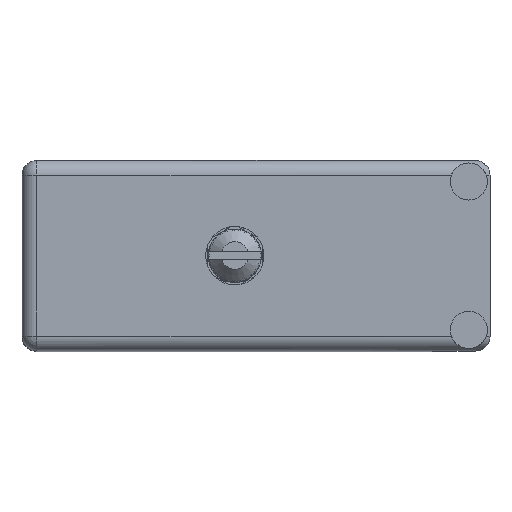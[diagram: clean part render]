
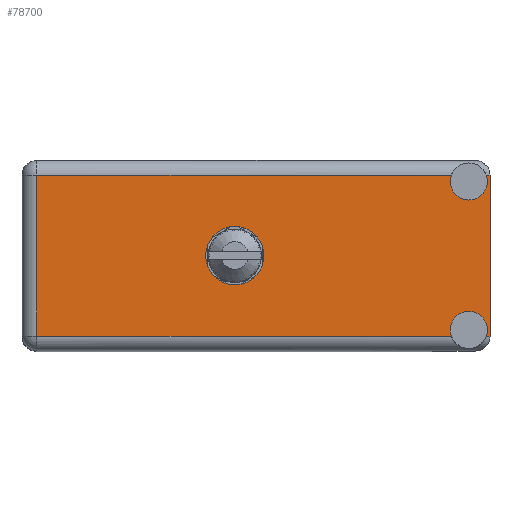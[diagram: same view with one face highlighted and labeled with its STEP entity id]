
A CAD part, top view. The second image highlights one B-rep face of the part: STEP entity #78700.
In plain terms, the highlighted face is planar.
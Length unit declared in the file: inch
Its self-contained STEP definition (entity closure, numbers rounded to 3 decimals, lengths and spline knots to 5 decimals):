
#2016 = EDGE_CURVE ( 'NONE', #110366, #90084, #36527, .T. ) ;
#2935 = CARTESIAN_POINT ( 'NONE',  ( 1.004, 1.566, -0.4495 ) ) ;
#3566 = CARTESIAN_POINT ( 'NONE',  ( 2.208, 1.566, -0.07 ) ) ;
#3950 = DIRECTION ( 'NONE',  ( 0., 1., 0. ) ) ;
#4356 = VERTEX_POINT ( 'NONE', #86213 ) ;
#5096 = ORIENTED_EDGE ( 'NONE', *, *, #92905, .T. ) ;
#5624 = EDGE_LOOP ( 'NONE', ( #109971, #22260, #44195, #107811, #81804, #33854, #102576, #89367, #27568, #5096 ) ) ;
#7193 = CARTESIAN_POINT ( 'NONE',  ( 2.19038, 1.566, -0.07 ) ) ;
#8008 = VERTEX_POINT ( 'NONE', #30675 ) ;
#9982 = CARTESIAN_POINT ( 'NONE',  ( 0., 1.566, -0.829 ) ) ;
#11879 = DIRECTION ( 'NONE',  ( 0., 0., 1. ) ) ;
#13929 = CARTESIAN_POINT ( 'NONE',  ( 0.07, 1.566, -0.07 ) ) ;
#14303 = VERTEX_POINT ( 'NONE', #78402 ) ;
#14353 = CARTESIAN_POINT ( 'NONE',  ( 2.208, 1.566, -0.07 ) ) ;
#14732 = VERTEX_POINT ( 'NONE', #71281 ) ;
#14805 = CARTESIAN_POINT ( 'NONE',  ( 0.07, 1.566, -0.829 ) ) ;
#18191 = CARTESIAN_POINT ( 'NONE',  ( 1.004, 1.566, -0.312 ) ) ;
#18658 = CIRCLE ( 'NONE', #94053, 0.0875 ) ;
#19000 = EDGE_CURVE ( 'NONE', #14303, #85294, #23795, .T. ) ;
#19820 = AXIS2_PLACEMENT_3D ( 'NONE', #71163, #61819, #53638 ) ;
#22245 = EDGE_CURVE ( 'NONE', #14732, #39829, #66998, .T. ) ;
#22260 = ORIENTED_EDGE ( 'NONE', *, *, #31615, .F. ) ;
#23795 = CIRCLE ( 'NONE', #19820, 0.1375 ) ;
#24312 = CIRCLE ( 'NONE', #114780, 0.0875 ) ;
#26989 = CARTESIAN_POINT ( 'NONE',  ( 2.108, 1.566, -0.0995 ) ) ;
#27568 = ORIENTED_EDGE ( 'NONE', *, *, #2016, .T. ) ;
#28002 = CARTESIAN_POINT ( 'NONE',  ( 2.108, 1.566, -0.0995 ) ) ;
#28774 = DIRECTION ( 'NONE',  ( 0., 0., 1. ) ) ;
#29146 = LINE ( 'NONE', #3566, #103081 ) ;
#29186 = EDGE_CURVE ( 'NONE', #110366, #4356, #18658, .T. ) ;
#30675 = CARTESIAN_POINT ( 'NONE',  ( 2.108, 1.566, -0.187 ) ) ;
#30737 = CARTESIAN_POINT ( 'NONE',  ( 2.02562, 1.566, -0.829 ) ) ;
#31615 = EDGE_CURVE ( 'NONE', #8008, #68920, #24312, .T. ) ;
#33402 = CARTESIAN_POINT ( 'NONE',  ( 2.02562, 1.566, -0.07 ) ) ;
#33520 = DIRECTION ( 'NONE',  ( 1., 0., 0. ) ) ;
#33854 = ORIENTED_EDGE ( 'NONE', *, *, #22245, .T. ) ;
#35209 = DIRECTION ( 'NONE',  ( 0., 0., 1. ) ) ;
#35634 = DIRECTION ( 'NONE',  ( -1., 0., 0. ) ) ;
#36142 = EDGE_LOOP ( 'NONE', ( #79937, #96858 ) ) ;
#36356 = CARTESIAN_POINT ( 'NONE',  ( 2.208, 1.566, 0. ) ) ;
#36527 = LINE ( 'NONE', #9982, #104851 ) ;
#38029 = LINE ( 'NONE', #82446, #76975 ) ;
#39829 = VERTEX_POINT ( 'NONE', #103362 ) ;
#44177 = CARTESIAN_POINT ( 'NONE',  ( 2.108, 1.566, -0.7995 ) ) ;
#44195 = ORIENTED_EDGE ( 'NONE', *, *, #73581, .F. ) ;
#48921 = LINE ( 'NONE', #61186, #107485 ) ;
#50059 = DIRECTION ( 'NONE',  ( 0., 0., 1. ) ) ;
#51718 = VECTOR ( 'NONE', #58402, 39.37008 ) ;
#53400 = CIRCLE ( 'NONE', #66712, 0.0875 ) ;
#53638 = DIRECTION ( 'NONE',  ( 0., 0., 1. ) ) ;
#53927 = DIRECTION ( 'NONE',  ( 0., 0., 1. ) ) ;
#58402 = DIRECTION ( 'NONE',  ( -1., 0., 0. ) ) ;
#58977 = CIRCLE ( 'NONE', #114504, 0.1375 ) ;
#59398 = DIRECTION ( 'NONE',  ( 0., 1., 0. ) ) ;
#61186 = CARTESIAN_POINT ( 'NONE',  ( 2.208, 1.566, -0.07 ) ) ;
#61330 = DIRECTION ( 'NONE',  ( 0., 0., 1. ) ) ;
#61819 = DIRECTION ( 'NONE',  ( 0., 1., 0. ) ) ;
#63246 = DIRECTION ( 'NONE',  ( 0., 1., 0. ) ) ;
#64933 = FACE_BOUND ( 'NONE', #36142, .T. ) ;
#66712 = AXIS2_PLACEMENT_3D ( 'NONE', #44177, #107260, #61330 ) ;
#66998 = LINE ( 'NONE', #109500, #51718 ) ;
#68920 = VERTEX_POINT ( 'NONE', #33402 ) ;
#70674 = DIRECTION ( 'NONE',  ( 0., 0., 1. ) ) ;
#71163 = CARTESIAN_POINT ( 'NONE',  ( 1.004, 1.566, -0.4495 ) ) ;
#71281 = CARTESIAN_POINT ( 'NONE',  ( 2.208, 1.566, -0.829 ) ) ;
#73581 = EDGE_CURVE ( 'NONE', #88315, #8008, #78982, .T. ) ;
#74115 = VERTEX_POINT ( 'NONE', #14353 ) ;
#76975 = VECTOR ( 'NONE', #81665, 39.37008 ) ;
#77280 = CARTESIAN_POINT ( 'NONE',  ( 0., 1.566, -0.899 ) ) ;
#78402 = CARTESIAN_POINT ( 'NONE',  ( 1.004, 1.566, -0.587 ) ) ;
#78700 = ADVANCED_FACE ( 'NONE', ( #64933, #99868 ), #111615, .T. ) ;
#78982 = CIRCLE ( 'NONE', #91266, 0.0875 ) ;
#79937 = ORIENTED_EDGE ( 'NONE', *, *, #109669, .F. ) ;
#80832 = AXIS2_PLACEMENT_3D ( 'NONE', #77280, #59398, #50059 ) ;
#81665 = DIRECTION ( 'NONE',  ( 0., 0., 1. ) ) ;
#81804 = ORIENTED_EDGE ( 'NONE', *, *, #109503, .F. ) ;
#82446 = CARTESIAN_POINT ( 'NONE',  ( 0.07, 1.566, -0.899 ) ) ;
#82676 = LINE ( 'NONE', #36356, #109188 ) ;
#85294 = VERTEX_POINT ( 'NONE', #18191 ) ;
#86073 = EDGE_CURVE ( 'NONE', #88315, #74115, #29146, .T. ) ;
#86213 = CARTESIAN_POINT ( 'NONE',  ( 2.108, 1.566, -0.712 ) ) ;
#88315 = VERTEX_POINT ( 'NONE', #7193 ) ;
#89157 = VERTEX_POINT ( 'NONE', #13929 ) ;
#89367 = ORIENTED_EDGE ( 'NONE', *, *, #29186, .F. ) ;
#90084 = VERTEX_POINT ( 'NONE', #14805 ) ;
#91266 = AXIS2_PLACEMENT_3D ( 'NONE', #28002, #3950, #28774 ) ;
#92905 = EDGE_CURVE ( 'NONE', #90084, #89157, #38029, .T. ) ;
#94053 = AXIS2_PLACEMENT_3D ( 'NONE', #106139, #106525, #35209 ) ;
#96858 = ORIENTED_EDGE ( 'NONE', *, *, #19000, .F. ) ;
#99868 = FACE_OUTER_BOUND ( 'NONE', #5624, .T. ) ;
#102576 = ORIENTED_EDGE ( 'NONE', *, *, #109515, .F. ) ;
#103081 = VECTOR ( 'NONE', #111746, 39.37008 ) ;
#103362 = CARTESIAN_POINT ( 'NONE',  ( 2.19038, 1.566, -0.829 ) ) ;
#103649 = EDGE_CURVE ( 'NONE', #89157, #68920, #48921, .T. ) ;
#104851 = VECTOR ( 'NONE', #35634, 39.37008 ) ;
#106139 = CARTESIAN_POINT ( 'NONE',  ( 2.108, 1.566, -0.7995 ) ) ;
#106525 = DIRECTION ( 'NONE',  ( 0., 1., 0. ) ) ;
#107260 = DIRECTION ( 'NONE',  ( 0., 1., 0. ) ) ;
#107485 = VECTOR ( 'NONE', #33520, 39.37008 ) ;
#107811 = ORIENTED_EDGE ( 'NONE', *, *, #86073, .T. ) ;
#109188 = VECTOR ( 'NONE', #70674, 39.37008 ) ;
#109500 = CARTESIAN_POINT ( 'NONE',  ( 0., 1.566, -0.829 ) ) ;
#109503 = EDGE_CURVE ( 'NONE', #14732, #74115, #82676, .T. ) ;
#109515 = EDGE_CURVE ( 'NONE', #4356, #39829, #53400, .T. ) ;
#109669 = EDGE_CURVE ( 'NONE', #85294, #14303, #58977, .T. ) ;
#109969 = DIRECTION ( 'NONE',  ( 0., 1., 0. ) ) ;
#109971 = ORIENTED_EDGE ( 'NONE', *, *, #103649, .T. ) ;
#110366 = VERTEX_POINT ( 'NONE', #30737 ) ;
#111615 = PLANE ( 'NONE',  #80832 ) ;
#111746 = DIRECTION ( 'NONE',  ( 1., 0., 0. ) ) ;
#114504 = AXIS2_PLACEMENT_3D ( 'NONE', #2935, #109969, #11879 ) ;
#114780 = AXIS2_PLACEMENT_3D ( 'NONE', #26989, #63246, #53927 ) ;
